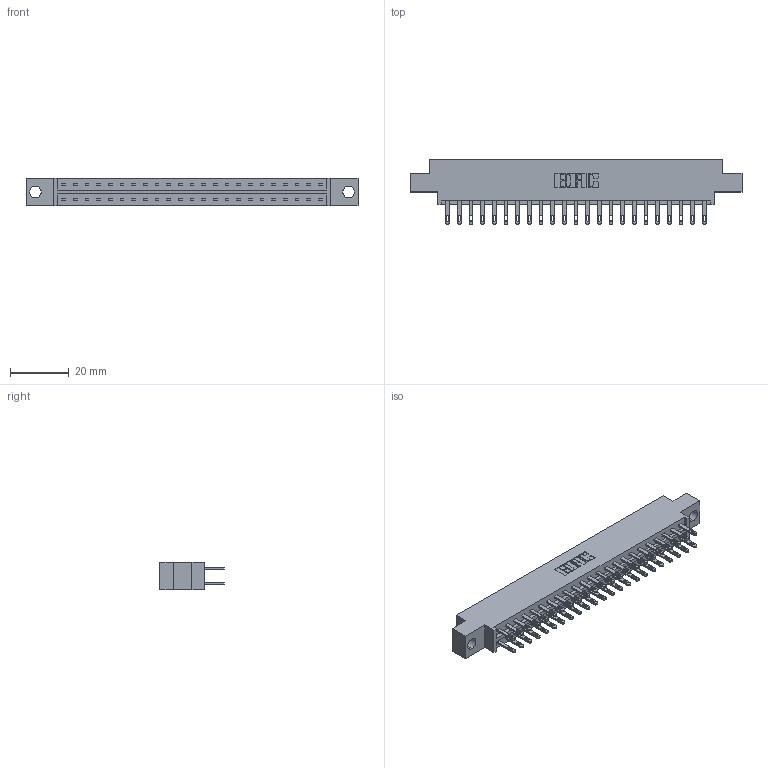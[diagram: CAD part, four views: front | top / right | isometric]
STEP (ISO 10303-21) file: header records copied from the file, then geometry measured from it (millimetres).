
FILE_DESCRIPTION (( 'STEP AP203' ), '1' );
FILE_NAME ('833-046-500-804.STEP', '2020-06-04T13:48:28', ( '' ), ( '' ), 'SwSTEP 2.0', 'SolidWorks 2020', '' );
FILE_SCHEMA (( 'CONFIG_CONTROL_DESIGN' ));
Length unit declared in the file: inch
Products named in the file (3): 833 Part_Offset - .156 Dia - TH; 833-046-500-804; 345-292-001_345-293-100
Assembly tree (47 placements, depth 2):
  833-046-500-804
    833 Part_Offset - .156 Dia - TH
    345-292-001_345-293-100  x46
Bounding box: 112.67 x 21.85 x 9.4 mm (x, y, z)
Volume: 11150.6 mm3; surface area: 13505.1 mm2
Topology: 47 solids, 47 shells, 2326 faces, 7085 edges, 4722 vertices
Faces by surface type: plane 1454, cylinder 872
Entity records: 17319 total; most frequent: CARTESIAN_POINT 2894, ORIENTED_EDGE 2830, DIRECTION 2507, EDGE_CURVE 1415, LINE 1283, VECTOR 1283, VERTEX_POINT 942, AXIS2_PLACEMENT_3D 612
